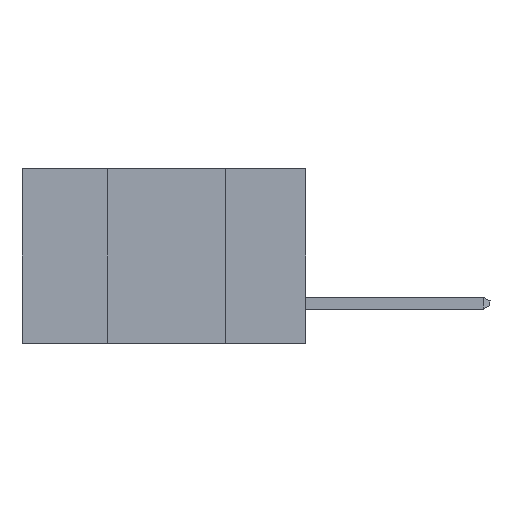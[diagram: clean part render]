
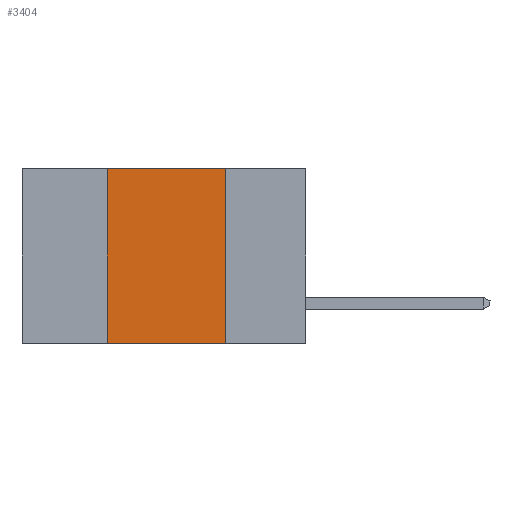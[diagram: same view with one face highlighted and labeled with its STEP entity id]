
A CAD part, left-side view. The second image highlights one B-rep face of the part: STEP entity #3404.
In plain terms, the highlighted planar face has unit normal (-1, 0, 0).
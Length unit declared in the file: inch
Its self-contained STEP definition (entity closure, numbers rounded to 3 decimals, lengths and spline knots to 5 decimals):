
#112 = VERTEX_POINT ( 'NONE', #443 ) ;
#227 = ORIENTED_EDGE ( 'NONE', *, *, #7733, .F. ) ;
#345 = DIRECTION ( 'NONE',  ( 0., 0., 1. ) ) ;
#443 = CARTESIAN_POINT ( 'NONE',  ( 0., 0.17, -0.37 ) ) ;
#489 = ORIENTED_EDGE ( 'NONE', *, *, #3091, .F. ) ;
#649 = EDGE_CURVE ( 'NONE', #6001, #6484, #10829, .T. ) ;
#1017 = CARTESIAN_POINT ( 'NONE',  ( 0., 0.17, -0.37 ) ) ;
#1578 = VERTEX_POINT ( 'NONE', #5617 ) ;
#1601 = ORIENTED_EDGE ( 'NONE', *, *, #649, .F. ) ;
#2034 = CARTESIAN_POINT ( 'NONE',  ( 0., 0.17, 0. ) ) ;
#2209 = CARTESIAN_POINT ( 'NONE',  ( 0., 0.42, -0.37 ) ) ;
#2709 = DIRECTION ( 'NONE',  ( 0., 0., -1. ) ) ;
#3081 = CARTESIAN_POINT ( 'NONE',  ( 0., 0.6, 0. ) ) ;
#3091 = EDGE_CURVE ( 'NONE', #6484, #112, #10868, .T. ) ;
#3352 = VECTOR ( 'NONE', #7640, 39.37008 ) ;
#3404 = ADVANCED_FACE ( 'NONE', ( #9618 ), #8798, .F. ) ;
#4290 = CARTESIAN_POINT ( 'NONE',  ( 0., 0.6, -0.37 ) ) ;
#4646 = DIRECTION ( 'NONE',  ( 1., 0., 0. ) ) ;
#5031 = VECTOR ( 'NONE', #6854, 39.37008 ) ;
#5617 = CARTESIAN_POINT ( 'NONE',  ( 0., 0.42, -0.37 ) ) ;
#6001 = VERTEX_POINT ( 'NONE', #7119 ) ;
#6050 = EDGE_LOOP ( 'NONE', ( #489, #1601, #227, #8862 ) ) ;
#6132 = CARTESIAN_POINT ( 'NONE',  ( 0., 0.6, 0. ) ) ;
#6484 = VERTEX_POINT ( 'NONE', #2034 ) ;
#6843 = AXIS2_PLACEMENT_3D ( 'NONE', #6132, #4646, #2709 ) ;
#6854 = DIRECTION ( 'NONE',  ( 0., -1., 0. ) ) ;
#7119 = CARTESIAN_POINT ( 'NONE',  ( 0., 0.42, 0. ) ) ;
#7640 = DIRECTION ( 'NONE',  ( 0., 0., -1. ) ) ;
#7733 = EDGE_CURVE ( 'NONE', #1578, #6001, #8723, .T. ) ;
#7868 = VECTOR ( 'NONE', #345, 39.37008 ) ;
#8723 = LINE ( 'NONE', #2209, #7868 ) ;
#8743 = VECTOR ( 'NONE', #9890, 39.37008 ) ;
#8798 = PLANE ( 'NONE',  #6843 ) ;
#8862 = ORIENTED_EDGE ( 'NONE', *, *, #8895, .T. ) ;
#8895 = EDGE_CURVE ( 'NONE', #1578, #112, #9319, .T. ) ;
#9319 = LINE ( 'NONE', #4290, #5031 ) ;
#9618 = FACE_OUTER_BOUND ( 'NONE', #6050, .T. ) ;
#9890 = DIRECTION ( 'NONE',  ( 0., -1., 0. ) ) ;
#10829 = LINE ( 'NONE', #3081, #8743 ) ;
#10868 = LINE ( 'NONE', #1017, #3352 ) ;
